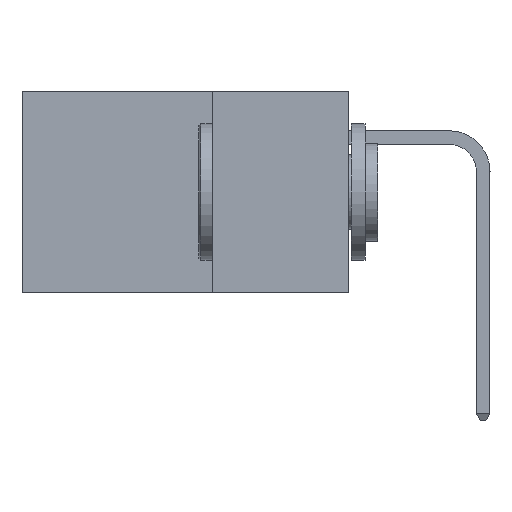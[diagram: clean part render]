
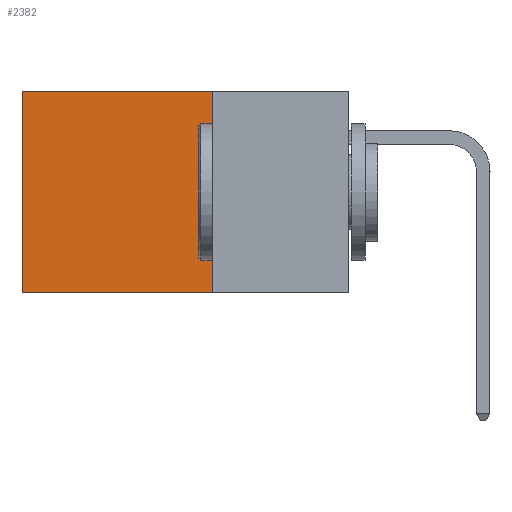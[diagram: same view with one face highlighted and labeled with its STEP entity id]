
A CAD part, left-side view. The second image highlights one B-rep face of the part: STEP entity #2382.
In plain terms, the highlighted planar face has unit normal (-1, 0, 0).
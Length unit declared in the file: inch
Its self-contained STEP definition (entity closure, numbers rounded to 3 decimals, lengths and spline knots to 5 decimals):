
#658 = CARTESIAN_POINT ( 'NONE',  ( 0.2875, 0.25, 0. ) ) ;
#1251 = CARTESIAN_POINT ( 'NONE',  ( 0.2875, 0.25, -0.37 ) ) ;
#2382 = ADVANCED_FACE ( 'NONE', ( #2746 ), #18032, .F. ) ;
#2746 = FACE_OUTER_BOUND ( 'NONE', #20023, .T. ) ;
#3059 = ORIENTED_EDGE ( 'NONE', *, *, #22268, .T. ) ;
#3208 = EDGE_CURVE ( 'NONE', #20064, #8744, #13949, .T. ) ;
#3939 = ORIENTED_EDGE ( 'NONE', *, *, #3208, .T. ) ;
#3947 = VECTOR ( 'NONE', #19427, 39.37008 ) ;
#4840 = VECTOR ( 'NONE', #23718, 39.37008 ) ;
#5531 = CARTESIAN_POINT ( 'NONE',  ( 0.2875, 0.25, 0. ) ) ;
#5800 = EDGE_CURVE ( 'NONE', #16907, #8744, #14865, .T. ) ;
#5842 = CARTESIAN_POINT ( 'NONE',  ( 0.2875, 0.25, 0. ) ) ;
#8291 = ORIENTED_EDGE ( 'NONE', *, *, #5800, .F. ) ;
#8380 = LINE ( 'NONE', #5842, #9578 ) ;
#8744 = VERTEX_POINT ( 'NONE', #13100 ) ;
#8811 = DIRECTION ( 'NONE',  ( 0., 0., -1. ) ) ;
#8993 = VECTOR ( 'NONE', #8811, 39.37008 ) ;
#9578 = VECTOR ( 'NONE', #18855, 39.37008 ) ;
#13100 = CARTESIAN_POINT ( 'NONE',  ( 0.2875, 0.6, -0.37 ) ) ;
#13424 = LINE ( 'NONE', #658, #3947 ) ;
#13555 = VERTEX_POINT ( 'NONE', #5531 ) ;
#13949 = LINE ( 'NONE', #21750, #8993 ) ;
#14865 = LINE ( 'NONE', #1251, #4840 ) ;
#15411 = ORIENTED_EDGE ( 'NONE', *, *, #16494, .F. ) ;
#16494 = EDGE_CURVE ( 'NONE', #13555, #16907, #8380, .T. ) ;
#16907 = VERTEX_POINT ( 'NONE', #20282 ) ;
#18032 = PLANE ( 'NONE',  #19805 ) ;
#18855 = DIRECTION ( 'NONE',  ( 0., 0., -1. ) ) ;
#19427 = DIRECTION ( 'NONE',  ( 0., 1., 0. ) ) ;
#19447 = CARTESIAN_POINT ( 'NONE',  ( 0.2875, 0.25, 0. ) ) ;
#19647 = DIRECTION ( 'NONE',  ( 1., 0., 0. ) ) ;
#19805 = AXIS2_PLACEMENT_3D ( 'NONE', #19447, #19647, #20446 ) ;
#20023 = EDGE_LOOP ( 'NONE', ( #3939, #8291, #15411, #3059 ) ) ;
#20064 = VERTEX_POINT ( 'NONE', #20163 ) ;
#20163 = CARTESIAN_POINT ( 'NONE',  ( 0.2875, 0.6, 0. ) ) ;
#20282 = CARTESIAN_POINT ( 'NONE',  ( 0.2875, 0.25, -0.37 ) ) ;
#20446 = DIRECTION ( 'NONE',  ( 0., 0., -1. ) ) ;
#21750 = CARTESIAN_POINT ( 'NONE',  ( 0.2875, 0.6, 0. ) ) ;
#22268 = EDGE_CURVE ( 'NONE', #13555, #20064, #13424, .T. ) ;
#23718 = DIRECTION ( 'NONE',  ( 0., 1., 0. ) ) ;
